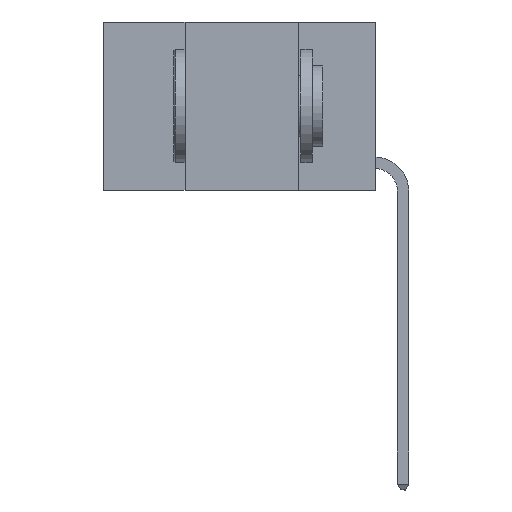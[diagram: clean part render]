
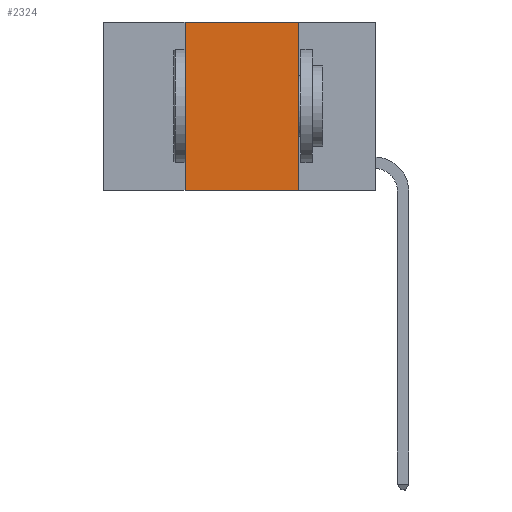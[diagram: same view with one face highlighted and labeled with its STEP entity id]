
A CAD part, left-side view. The second image highlights one B-rep face of the part: STEP entity #2324.
In plain terms, the highlighted planar face has unit normal (-1, 0, 0).
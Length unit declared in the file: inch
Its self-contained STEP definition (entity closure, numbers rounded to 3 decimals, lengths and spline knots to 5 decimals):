
#961 = CARTESIAN_POINT ( 'NONE',  ( 0., 0.6, -0.37 ) ) ;
#1032 = LINE ( 'NONE', #961, #13421 ) ;
#1048 = ORIENTED_EDGE ( 'NONE', *, *, #14141, .T. ) ;
#2135 = DIRECTION ( 'NONE',  ( 0., 0., 1. ) ) ;
#2324 = ADVANCED_FACE ( 'NONE', ( #12455 ), #9888, .F. ) ;
#2409 = AXIS2_PLACEMENT_3D ( 'NONE', #14741, #8923, #2818 ) ;
#2818 = DIRECTION ( 'NONE',  ( 0., 0., -1. ) ) ;
#5497 = ORIENTED_EDGE ( 'NONE', *, *, #12728, .F. ) ;
#5752 = CARTESIAN_POINT ( 'NONE',  ( 0., 0.17, 0. ) ) ;
#6053 = CARTESIAN_POINT ( 'NONE',  ( 0., 0.17, 0. ) ) ;
#6630 = ORIENTED_EDGE ( 'NONE', *, *, #6845, .F. ) ;
#6845 = EDGE_CURVE ( 'NONE', #8100, #7573, #6943, .T. ) ;
#6943 = LINE ( 'NONE', #5752, #15161 ) ;
#7573 = VERTEX_POINT ( 'NONE', #12722 ) ;
#7912 = VERTEX_POINT ( 'NONE', #11277 ) ;
#8100 = VERTEX_POINT ( 'NONE', #6053 ) ;
#8603 = LINE ( 'NONE', #13530, #13591 ) ;
#8923 = DIRECTION ( 'NONE',  ( 1., 0., 0. ) ) ;
#9131 = CARTESIAN_POINT ( 'NONE',  ( 0., 0.42, 0. ) ) ;
#9229 = VERTEX_POINT ( 'NONE', #11372 ) ;
#9299 = DIRECTION ( 'NONE',  ( 0., -1., 0. ) ) ;
#9361 = LINE ( 'NONE', #9131, #14814 ) ;
#9888 = PLANE ( 'NONE',  #2409 ) ;
#11277 = CARTESIAN_POINT ( 'NONE',  ( 0., 0.42, -0.37 ) ) ;
#11372 = CARTESIAN_POINT ( 'NONE',  ( 0., 0.42, 0. ) ) ;
#11895 = DIRECTION ( 'NONE',  ( 0., 0., -1. ) ) ;
#12074 = EDGE_LOOP ( 'NONE', ( #6630, #5497, #12855, #1048 ) ) ;
#12371 = DIRECTION ( 'NONE',  ( 0., -1., 0. ) ) ;
#12455 = FACE_OUTER_BOUND ( 'NONE', #12074, .T. ) ;
#12722 = CARTESIAN_POINT ( 'NONE',  ( 0., 0.17, -0.37 ) ) ;
#12728 = EDGE_CURVE ( 'NONE', #9229, #8100, #8603, .T. ) ;
#12855 = ORIENTED_EDGE ( 'NONE', *, *, #14489, .F. ) ;
#13421 = VECTOR ( 'NONE', #9299, 39.37008 ) ;
#13530 = CARTESIAN_POINT ( 'NONE',  ( 0., 0.6, 0. ) ) ;
#13591 = VECTOR ( 'NONE', #12371, 39.37008 ) ;
#14141 = EDGE_CURVE ( 'NONE', #7912, #7573, #1032, .T. ) ;
#14489 = EDGE_CURVE ( 'NONE', #7912, #9229, #9361, .T. ) ;
#14741 = CARTESIAN_POINT ( 'NONE',  ( 0., 0.6, 0. ) ) ;
#14814 = VECTOR ( 'NONE', #2135, 39.37008 ) ;
#15161 = VECTOR ( 'NONE', #11895, 39.37008 ) ;
